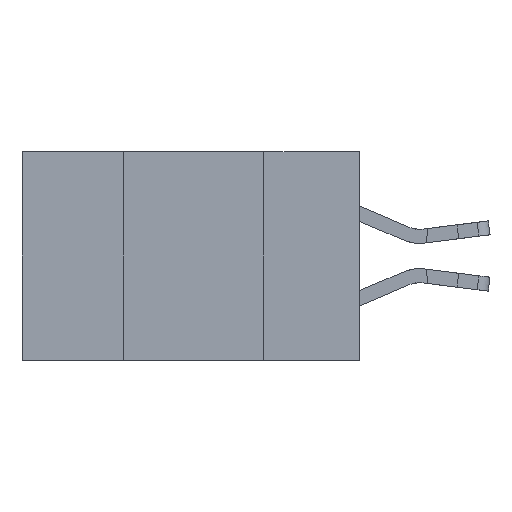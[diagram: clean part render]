
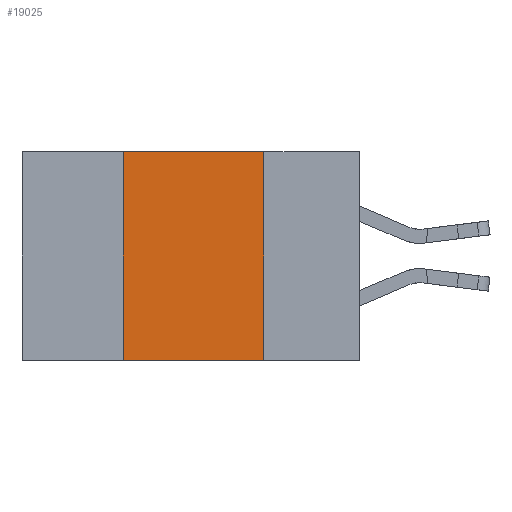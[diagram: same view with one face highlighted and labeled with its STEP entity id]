
A CAD part, left-side view. The second image highlights one B-rep face of the part: STEP entity #19025.
In plain terms, the highlighted planar face has unit normal (-1, 0, 0).
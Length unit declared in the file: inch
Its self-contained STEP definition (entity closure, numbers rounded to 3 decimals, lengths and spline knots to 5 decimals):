
#821 = CARTESIAN_POINT ( 'NONE',  ( 0., 0.6, 0. ) ) ;
#822 = PLANE ( 'NONE',  #24776 ) ;
#3043 = LINE ( 'NONE', #7190, #4341 ) ;
#3133 = ORIENTED_EDGE ( 'NONE', *, *, #17250, .F. ) ;
#3484 = LINE ( 'NONE', #821, #13807 ) ;
#4341 = VECTOR ( 'NONE', #13339, 39.37008 ) ;
#4710 = ORIENTED_EDGE ( 'NONE', *, *, #15578, .F. ) ;
#5913 = ORIENTED_EDGE ( 'NONE', *, *, #10727, .T. ) ;
#6050 = EDGE_CURVE ( 'NONE', #15651, #25235, #3484, .T. ) ;
#7190 = CARTESIAN_POINT ( 'NONE',  ( 0., 0.17, 0. ) ) ;
#7394 = CARTESIAN_POINT ( 'NONE',  ( 0., 0.17, -0.37 ) ) ;
#8979 = VECTOR ( 'NONE', #18626, 39.37008 ) ;
#9801 = CARTESIAN_POINT ( 'NONE',  ( 0., 0.42, 0. ) ) ;
#9804 = CARTESIAN_POINT ( 'NONE',  ( 0., 0.42, -0.37 ) ) ;
#10292 = CARTESIAN_POINT ( 'NONE',  ( 0., 0.6, -0.37 ) ) ;
#10727 = EDGE_CURVE ( 'NONE', #24005, #25341, #21521, .T. ) ;
#12602 = FACE_OUTER_BOUND ( 'NONE', #21510, .T. ) ;
#13339 = DIRECTION ( 'NONE',  ( 0., 0., -1. ) ) ;
#13807 = VECTOR ( 'NONE', #17517, 39.37008 ) ;
#15578 = EDGE_CURVE ( 'NONE', #24005, #15651, #15754, .T. ) ;
#15651 = VERTEX_POINT ( 'NONE', #9801 ) ;
#15721 = ORIENTED_EDGE ( 'NONE', *, *, #6050, .F. ) ;
#15754 = LINE ( 'NONE', #22789, #8979 ) ;
#17243 = VECTOR ( 'NONE', #24999, 39.37008 ) ;
#17250 = EDGE_CURVE ( 'NONE', #25235, #25341, #3043, .T. ) ;
#17517 = DIRECTION ( 'NONE',  ( 0., -1., 0. ) ) ;
#17519 = DIRECTION ( 'NONE',  ( 1., 0., 0. ) ) ;
#18626 = DIRECTION ( 'NONE',  ( 0., 0., 1. ) ) ;
#19025 = ADVANCED_FACE ( 'NONE', ( #12602 ), #822, .F. ) ;
#21510 = EDGE_LOOP ( 'NONE', ( #3133, #15721, #4710, #5913 ) ) ;
#21521 = LINE ( 'NONE', #10292, #17243 ) ;
#21745 = CARTESIAN_POINT ( 'NONE',  ( 0., 0.17, 0. ) ) ;
#22789 = CARTESIAN_POINT ( 'NONE',  ( 0., 0.42, 0. ) ) ;
#23715 = CARTESIAN_POINT ( 'NONE',  ( 0., 0.6, 0. ) ) ;
#24005 = VERTEX_POINT ( 'NONE', #9804 ) ;
#24776 = AXIS2_PLACEMENT_3D ( 'NONE', #23715, #17519, #25545 ) ;
#24999 = DIRECTION ( 'NONE',  ( 0., -1., 0. ) ) ;
#25235 = VERTEX_POINT ( 'NONE', #21745 ) ;
#25341 = VERTEX_POINT ( 'NONE', #7394 ) ;
#25545 = DIRECTION ( 'NONE',  ( 0., 0., -1. ) ) ;
